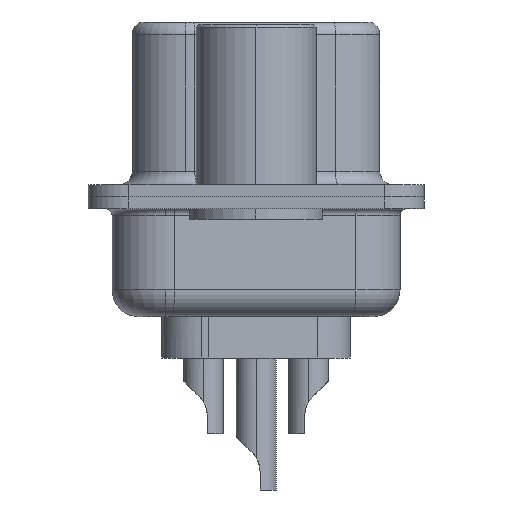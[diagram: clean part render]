
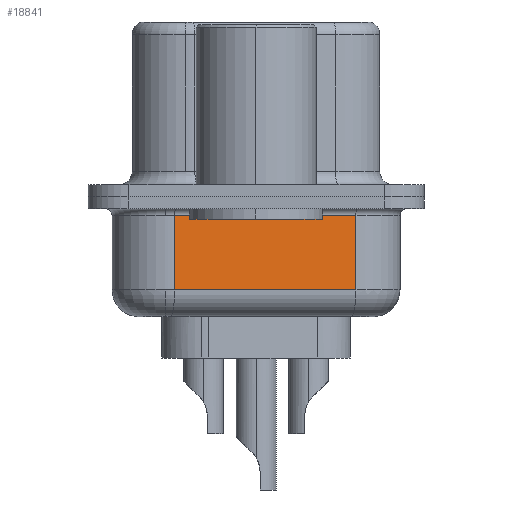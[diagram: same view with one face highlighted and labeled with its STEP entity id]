
A CAD part, left-side view. The second image highlights one B-rep face of the part: STEP entity #18841.
In plain terms, the highlighted planar face has unit normal (-0.985, -0.174, 0).
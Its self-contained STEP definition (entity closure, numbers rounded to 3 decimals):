
#609 = ORIENTED_EDGE ( 'NONE', *, *, #8503, .T. ) ;
#1087 = DIRECTION ( 'NONE',  ( -0.174, 0.985, 0. ) ) ;
#2084 = CARTESIAN_POINT ( 'NONE',  ( 4.124, -3.747, -0.7 ) ) ;
#2583 = ORIENTED_EDGE ( 'NONE', *, *, #4351, .F. ) ;
#3137 = CARTESIAN_POINT ( 'NONE',  ( 4.124, -3.747, -3.5 ) ) ;
#3165 = DIRECTION ( 'NONE',  ( 0.985, 0.174, 0. ) ) ;
#4058 = CARTESIAN_POINT ( 'NONE',  ( 2.925, 3.053, -0.7 ) ) ;
#4351 = EDGE_CURVE ( 'NONE', #7775, #11471, #7407, .T. ) ;
#5529 = VERTEX_POINT ( 'NONE', #2084 ) ;
#5941 = FACE_OUTER_BOUND ( 'NONE', #17184, .T. ) ;
#6046 = VECTOR ( 'NONE', #13816, 1000. ) ;
#6140 = EDGE_CURVE ( 'NONE', #10115, #5529, #6357, .T. ) ;
#6357 = LINE ( 'NONE', #12749, #15561 ) ;
#7407 = LINE ( 'NONE', #18664, #6046 ) ;
#7775 = VERTEX_POINT ( 'NONE', #14506 ) ;
#8103 = DIRECTION ( 'NONE',  ( 0., 0., 1. ) ) ;
#8503 = EDGE_CURVE ( 'NONE', #5529, #11471, #11867, .T. ) ;
#9107 = LINE ( 'NONE', #13860, #17979 ) ;
#9396 = CARTESIAN_POINT ( 'NONE',  ( 2.925, 3.053, -0.7 ) ) ;
#10115 = VERTEX_POINT ( 'NONE', #3137 ) ;
#10133 = ORIENTED_EDGE ( 'NONE', *, *, #17799, .T. ) ;
#11471 = VERTEX_POINT ( 'NONE', #9396 ) ;
#11784 = DIRECTION ( 'NONE',  ( 0.174, -0.985, 0. ) ) ;
#11867 = LINE ( 'NONE', #4058, #12709 ) ;
#12709 = VECTOR ( 'NONE', #1087, 1000. ) ;
#12749 = CARTESIAN_POINT ( 'NONE',  ( 4.124, -3.747, -4.5 ) ) ;
#13228 = ORIENTED_EDGE ( 'NONE', *, *, #6140, .T. ) ;
#13816 = DIRECTION ( 'NONE',  ( 0., 0., 1. ) ) ;
#13860 = CARTESIAN_POINT ( 'NONE',  ( 2.925, 3.053, -3.5 ) ) ;
#13986 = PLANE ( 'NONE',  #20222 ) ;
#14506 = CARTESIAN_POINT ( 'NONE',  ( 2.925, 3.053, -3.5 ) ) ;
#15561 = VECTOR ( 'NONE', #8103, 1000. ) ;
#16979 = CARTESIAN_POINT ( 'NONE',  ( 2.925, 3.053, -4.5 ) ) ;
#17184 = EDGE_LOOP ( 'NONE', ( #2583, #10133, #13228, #609 ) ) ;
#17799 = EDGE_CURVE ( 'NONE', #7775, #10115, #9107, .T. ) ;
#17979 = VECTOR ( 'NONE', #11784, 1000. ) ;
#18664 = CARTESIAN_POINT ( 'NONE',  ( 2.925, 3.053, -4.5 ) ) ;
#18736 = DIRECTION ( 'NONE',  ( -0.174, 0.985, 0. ) ) ;
#18841 = ADVANCED_FACE ( 'NONE', ( #5941 ), #13986, .F. ) ;
#20222 = AXIS2_PLACEMENT_3D ( 'NONE', #16979, #3165, #18736 ) ;
